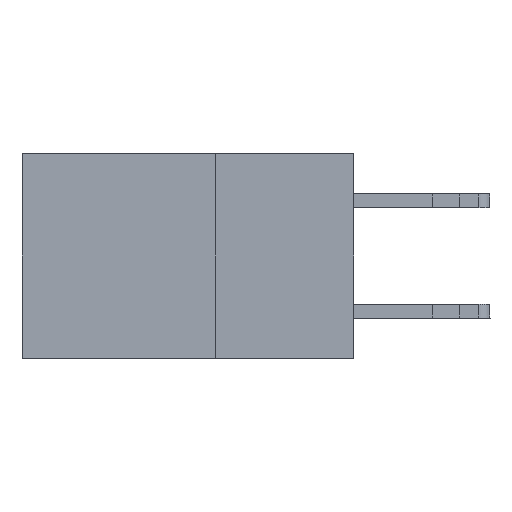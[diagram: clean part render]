
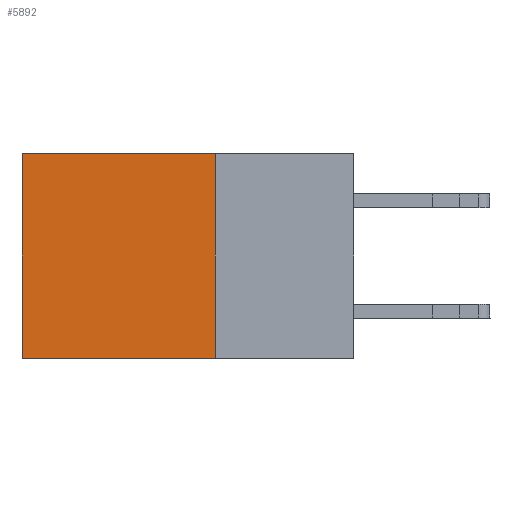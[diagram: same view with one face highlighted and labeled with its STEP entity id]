
A CAD part, left-side view. The second image highlights one B-rep face of the part: STEP entity #5892.
In plain terms, the highlighted planar face has unit normal (-1, 0, 0).
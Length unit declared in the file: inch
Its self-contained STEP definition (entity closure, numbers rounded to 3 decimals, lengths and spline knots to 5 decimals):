
#510 = DIRECTION ( 'NONE',  ( 0., 1., 0. ) ) ;
#1246 = CARTESIAN_POINT ( 'NONE',  ( 0.2875, 0.25, -0.37 ) ) ;
#1994 = AXIS2_PLACEMENT_3D ( 'NONE', #13770, #3618, #15479 ) ;
#2627 = ORIENTED_EDGE ( 'NONE', *, *, #21201, .T. ) ;
#3618 = DIRECTION ( 'NONE',  ( 1., 0., 0. ) ) ;
#3813 = VERTEX_POINT ( 'NONE', #10949 ) ;
#4907 = VERTEX_POINT ( 'NONE', #9419 ) ;
#4921 = LINE ( 'NONE', #19057, #13418 ) ;
#5892 = ADVANCED_FACE ( 'NONE', ( #17512 ), #12059, .F. ) ;
#6600 = LINE ( 'NONE', #1246, #18451 ) ;
#7136 = CARTESIAN_POINT ( 'NONE',  ( 0.2875, 0.6, 0. ) ) ;
#8855 = VERTEX_POINT ( 'NONE', #13329 ) ;
#9165 = ORIENTED_EDGE ( 'NONE', *, *, #20871, .F. ) ;
#9419 = CARTESIAN_POINT ( 'NONE',  ( 0.2875, 0.25, 0. ) ) ;
#9854 = EDGE_CURVE ( 'NONE', #4907, #16738, #4921, .T. ) ;
#10334 = CARTESIAN_POINT ( 'NONE',  ( 0.2875, 0.25, -0.37 ) ) ;
#10650 = CARTESIAN_POINT ( 'NONE',  ( 0.2875, 0.25, 0. ) ) ;
#10949 = CARTESIAN_POINT ( 'NONE',  ( 0.2875, 0.6, -0.37 ) ) ;
#11095 = ORIENTED_EDGE ( 'NONE', *, *, #9854, .F. ) ;
#11357 = DIRECTION ( 'NONE',  ( 0., 1., 0. ) ) ;
#12059 = PLANE ( 'NONE',  #1994 ) ;
#12446 = VECTOR ( 'NONE', #17236, 39.37008 ) ;
#13329 = CARTESIAN_POINT ( 'NONE',  ( 0.2875, 0.6, 0. ) ) ;
#13418 = VECTOR ( 'NONE', #15805, 39.37008 ) ;
#13770 = CARTESIAN_POINT ( 'NONE',  ( 0.2875, 0.25, 0. ) ) ;
#14048 = ORIENTED_EDGE ( 'NONE', *, *, #19672, .T. ) ;
#15479 = DIRECTION ( 'NONE',  ( 0., 0., -1. ) ) ;
#15805 = DIRECTION ( 'NONE',  ( 0., 0., -1. ) ) ;
#16738 = VERTEX_POINT ( 'NONE', #10334 ) ;
#16929 = LINE ( 'NONE', #7136, #12446 ) ;
#16966 = LINE ( 'NONE', #10650, #20837 ) ;
#17236 = DIRECTION ( 'NONE',  ( 0., 0., -1. ) ) ;
#17512 = FACE_OUTER_BOUND ( 'NONE', #19707, .T. ) ;
#18451 = VECTOR ( 'NONE', #11357, 39.37008 ) ;
#19057 = CARTESIAN_POINT ( 'NONE',  ( 0.2875, 0.25, 0. ) ) ;
#19672 = EDGE_CURVE ( 'NONE', #4907, #8855, #16966, .T. ) ;
#19707 = EDGE_LOOP ( 'NONE', ( #2627, #9165, #11095, #14048 ) ) ;
#20837 = VECTOR ( 'NONE', #510, 39.37008 ) ;
#20871 = EDGE_CURVE ( 'NONE', #16738, #3813, #6600, .T. ) ;
#21201 = EDGE_CURVE ( 'NONE', #8855, #3813, #16929, .T. ) ;
